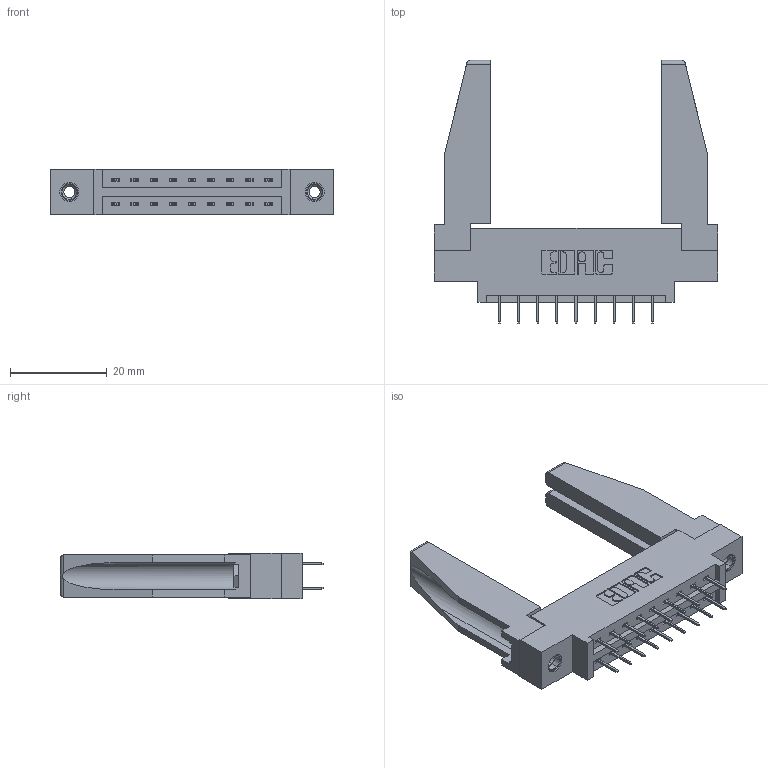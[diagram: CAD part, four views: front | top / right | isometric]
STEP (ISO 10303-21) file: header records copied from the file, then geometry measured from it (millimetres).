
FILE_DESCRIPTION (( 'STEP AP203' ), '1' );
FILE_NAME ('387-018-524-878.STEP', '2019-10-16T01:00:16', ( '' ), ( '' ), 'SwSTEP 2.0', 'SolidWorks 2016', '' );
FILE_SCHEMA (( 'CONFIG_CONTROL_DESIGN' ));
Length unit declared in the file: inch
Products named in the file (5): 337 Part_0.170 Offset - 0.156 Dia-TI; 345-250-001_345-250-001-102; 345-292-001_345-293-124; 307-220-078; 387-018-524-878
Assembly tree (23 placements, depth 2):
  387-018-524-878
    337 Part_0.170 Offset - 0.156 Dia-TI
    345-292-001_345-293-124  x18
    345-250-001_345-250-001-102  x2
    307-220-078  x2
Bounding box: 58.67 x 54.49 x 9.4 mm (x, y, z)
Volume: 9592.9 mm3; surface area: 9863.7 mm2
Topology: 23 solids, 23 shells, 1292 faces, 3623 edges, 2334 vertices
Faces by surface type: plane 950, cylinder 326, cone 12, torus 4
Entity records: 13892 total; most frequent: CARTESIAN_POINT 2368, ORIENTED_EDGE 2260, DIRECTION 2082, EDGE_CURVE 1130, VECTOR 968, LINE 968, VERTEX_POINT 744, AXIS2_PLACEMENT_3D 557
